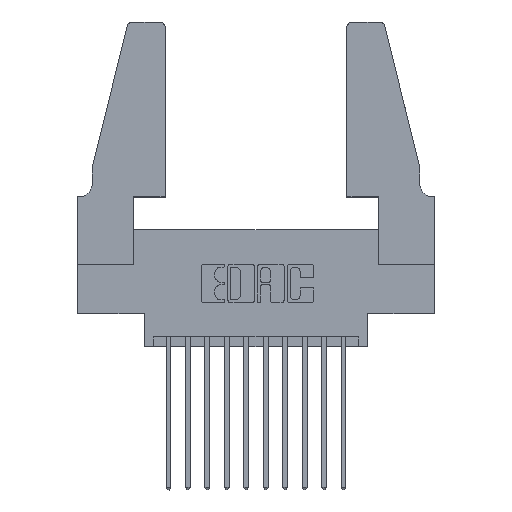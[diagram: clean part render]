
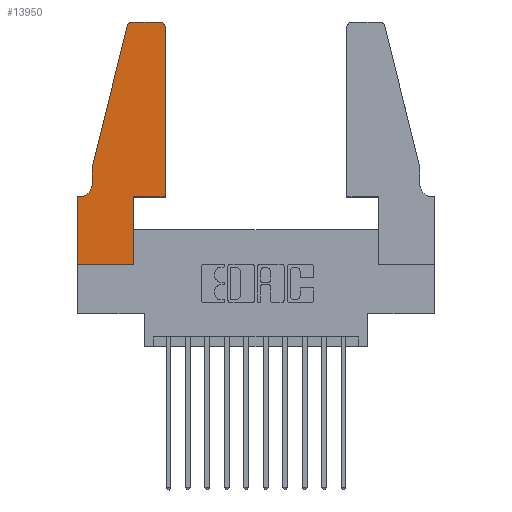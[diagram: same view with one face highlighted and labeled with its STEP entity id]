
A CAD part, top view. The second image highlights one B-rep face of the part: STEP entity #13950.
In plain terms, the highlighted planar face has unit normal (0, 0, 1).
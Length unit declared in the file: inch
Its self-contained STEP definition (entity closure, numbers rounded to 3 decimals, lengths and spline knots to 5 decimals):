
#338 = EDGE_CURVE ( 'NONE', #12182, #7786, #9535, .T. ) ;
#450 = CARTESIAN_POINT ( 'NONE',  ( 0., 0., 0.37 ) ) ;
#765 = VECTOR ( 'NONE', #12722, 39.37008 ) ;
#944 = ORIENTED_EDGE ( 'NONE', *, *, #14025, .T. ) ;
#970 = LINE ( 'NONE', #11142, #13198 ) ;
#1076 = ORIENTED_EDGE ( 'NONE', *, *, #338, .T. ) ;
#1112 = LINE ( 'NONE', #12904, #765 ) ;
#1614 = ORIENTED_EDGE ( 'NONE', *, *, #1717, .T. ) ;
#1717 = EDGE_CURVE ( 'NONE', #2778, #13175, #6778, .T. ) ;
#1848 = CARTESIAN_POINT ( 'NONE',  ( 0.2605, 1.25, 0.37 ) ) ;
#2038 = CARTESIAN_POINT ( 'NONE',  ( 0.0755, 0.5, 0.37 ) ) ;
#2198 = CARTESIAN_POINT ( 'NONE',  ( 0.0755, 0.42, 0.37 ) ) ;
#2309 = VERTEX_POINT ( 'NONE', #2038 ) ;
#2341 = CARTESIAN_POINT ( 'NONE',  ( 0., 0.35, 0.37 ) ) ;
#2718 = DIRECTION ( 'NONE',  ( 0., -1., 0. ) ) ;
#2744 = DIRECTION ( 'NONE',  ( -1., 0., 0. ) ) ;
#2778 = VERTEX_POINT ( 'NONE', #10514 ) ;
#2818 = CARTESIAN_POINT ( 'NONE',  ( 0., 0., 0.37 ) ) ;
#2894 = ORIENTED_EDGE ( 'NONE', *, *, #13201, .T. ) ;
#3040 = VERTEX_POINT ( 'NONE', #12127 ) ;
#3159 = AXIS2_PLACEMENT_3D ( 'NONE', #13959, #9419, #2744 ) ;
#3194 = LINE ( 'NONE', #6531, #11708 ) ;
#3258 = CARTESIAN_POINT ( 'NONE',  ( 0.0055, 0.35, 0.37 ) ) ;
#3302 = DIRECTION ( 'NONE',  ( -1., 0., 0. ) ) ;
#3457 = DIRECTION ( 'NONE',  ( 0., 0., 1. ) ) ;
#3555 = DIRECTION ( 'NONE',  ( 0., 0., 1. ) ) ;
#3777 = DIRECTION ( 'NONE',  ( 1., 0., 0. ) ) ;
#4109 = LINE ( 'NONE', #12534, #6347 ) ;
#4154 = VECTOR ( 'NONE', #7382, 39.37008 ) ;
#4204 = CARTESIAN_POINT ( 'NONE',  ( 0.2865, 0.35, 0.37 ) ) ;
#4251 = LINE ( 'NONE', #450, #8749 ) ;
#4361 = VERTEX_POINT ( 'NONE', #9597 ) ;
#4461 = CARTESIAN_POINT ( 'NONE',  ( 0.25487, 1.22718, 0.37 ) ) ;
#4660 = AXIS2_PLACEMENT_3D ( 'NONE', #10154, #3457, #11219 ) ;
#4676 = EDGE_CURVE ( 'NONE', #10553, #12045, #11576, .T. ) ;
#5004 = FACE_OUTER_BOUND ( 'NONE', #14251, .T. ) ;
#5472 = CARTESIAN_POINT ( 'NONE',  ( 0.284, 1.22, 0.37 ) ) ;
#5544 = ORIENTED_EDGE ( 'NONE', *, *, #4676, .T. ) ;
#5719 = ORIENTED_EDGE ( 'NONE', *, *, #8853, .T. ) ;
#6009 = DIRECTION ( 'NONE',  ( 1., 0., 0. ) ) ;
#6039 = DIRECTION ( 'NONE',  ( 0., -1., 0. ) ) ;
#6179 = VECTOR ( 'NONE', #3777, 39.37008 ) ;
#6347 = VECTOR ( 'NONE', #6039, 39.37008 ) ;
#6531 = CARTESIAN_POINT ( 'NONE',  ( 0.0755, 0.35, 0.37 ) ) ;
#6666 = AXIS2_PLACEMENT_3D ( 'NONE', #2341, #3555, #6862 ) ;
#6708 = DIRECTION ( 'NONE',  ( -0.239, -0.971, 0. ) ) ;
#6778 = CIRCLE ( 'NONE', #11826, 0.03 ) ;
#6862 = DIRECTION ( 'NONE',  ( 1., 0., 0. ) ) ;
#6873 = EDGE_CURVE ( 'NONE', #3040, #7133, #4251, .T. ) ;
#7133 = VERTEX_POINT ( 'NONE', #2818 ) ;
#7382 = DIRECTION ( 'NONE',  ( -1., 0., 0. ) ) ;
#7710 = DIRECTION ( 'NONE',  ( 0., 0., 1. ) ) ;
#7786 = VERTEX_POINT ( 'NONE', #3258 ) ;
#7828 = EDGE_CURVE ( 'NONE', #12045, #11913, #1112, .T. ) ;
#8384 = VERTEX_POINT ( 'NONE', #13131 ) ;
#8546 = LINE ( 'NONE', #1848, #4154 ) ;
#8749 = VECTOR ( 'NONE', #2718, 39.37008 ) ;
#8824 = ORIENTED_EDGE ( 'NONE', *, *, #6873, .T. ) ;
#8853 = EDGE_CURVE ( 'NONE', #2309, #12182, #4109, .T. ) ;
#8856 = ORIENTED_EDGE ( 'NONE', *, *, #9802, .T. ) ;
#9352 = CARTESIAN_POINT ( 'NONE',  ( 0.4505, 0.35, 0.37 ) ) ;
#9419 = DIRECTION ( 'NONE',  ( 0., 0., -1. ) ) ;
#9535 = CIRCLE ( 'NONE', #3159, 0.07 ) ;
#9597 = CARTESIAN_POINT ( 'NONE',  ( 0.4205, 1.25, 0.37 ) ) ;
#9599 = VECTOR ( 'NONE', #14372, 39.37008 ) ;
#9756 = VECTOR ( 'NONE', #14458, 39.37008 ) ;
#9802 = EDGE_CURVE ( 'NONE', #7786, #3040, #3194, .T. ) ;
#10154 = CARTESIAN_POINT ( 'NONE',  ( 0.4205, 1.22, 0.37 ) ) ;
#10514 = CARTESIAN_POINT ( 'NONE',  ( 0.284, 1.25, 0.37 ) ) ;
#10553 = VERTEX_POINT ( 'NONE', #14021 ) ;
#10754 = EDGE_CURVE ( 'NONE', #8384, #10553, #12530, .T. ) ;
#10762 = ORIENTED_EDGE ( 'NONE', *, *, #7828, .T. ) ;
#10914 = ORIENTED_EDGE ( 'NONE', *, *, #12144, .T. ) ;
#11142 = CARTESIAN_POINT ( 'NONE',  ( 0.0755, 0.5, 0.37 ) ) ;
#11219 = DIRECTION ( 'NONE',  ( 1., 0., 0. ) ) ;
#11576 = LINE ( 'NONE', #9352, #6179 ) ;
#11708 = VECTOR ( 'NONE', #3302, 39.37008 ) ;
#11826 = AXIS2_PLACEMENT_3D ( 'NONE', #5472, #7710, #6009 ) ;
#11830 = LINE ( 'NONE', #14369, #9756 ) ;
#11913 = VERTEX_POINT ( 'NONE', #11950 ) ;
#11950 = CARTESIAN_POINT ( 'NONE',  ( 0.4505, 1.22, 0.37 ) ) ;
#11962 = CIRCLE ( 'NONE', #4660, 0.03 ) ;
#12045 = VERTEX_POINT ( 'NONE', #13213 ) ;
#12112 = ORIENTED_EDGE ( 'NONE', *, *, #10754, .T. ) ;
#12127 = CARTESIAN_POINT ( 'NONE',  ( 0., 0.35, 0.37 ) ) ;
#12144 = EDGE_CURVE ( 'NONE', #7133, #8384, #11830, .T. ) ;
#12182 = VERTEX_POINT ( 'NONE', #2198 ) ;
#12298 = ORIENTED_EDGE ( 'NONE', *, *, #13777, .T. ) ;
#12530 = LINE ( 'NONE', #4204, #9599 ) ;
#12534 = CARTESIAN_POINT ( 'NONE',  ( 0.0755, 0.5, 0.37 ) ) ;
#12722 = DIRECTION ( 'NONE',  ( 0., 1., 0. ) ) ;
#12904 = CARTESIAN_POINT ( 'NONE',  ( 0.4505, 0.35, 0.37 ) ) ;
#13131 = CARTESIAN_POINT ( 'NONE',  ( 0.2865, 0., 0.37 ) ) ;
#13175 = VERTEX_POINT ( 'NONE', #4461 ) ;
#13198 = VECTOR ( 'NONE', #6708, 39.37008 ) ;
#13201 = EDGE_CURVE ( 'NONE', #13175, #2309, #970, .T. ) ;
#13213 = CARTESIAN_POINT ( 'NONE',  ( 0.4505, 0.35, 0.37 ) ) ;
#13500 = PLANE ( 'NONE',  #6666 ) ;
#13777 = EDGE_CURVE ( 'NONE', #4361, #2778, #8546, .T. ) ;
#13950 = ADVANCED_FACE ( 'NONE', ( #5004 ), #13500, .T. ) ;
#13959 = CARTESIAN_POINT ( 'NONE',  ( 0.0055, 0.42, 0.37 ) ) ;
#14021 = CARTESIAN_POINT ( 'NONE',  ( 0.2865, 0.35, 0.37 ) ) ;
#14025 = EDGE_CURVE ( 'NONE', #11913, #4361, #11962, .T. ) ;
#14251 = EDGE_LOOP ( 'NONE', ( #12298, #1614, #2894, #5719, #1076, #8856, #8824, #10914, #12112, #5544, #10762, #944 ) ) ;
#14369 = CARTESIAN_POINT ( 'NONE',  ( 0., 0., 0.37 ) ) ;
#14372 = DIRECTION ( 'NONE',  ( 0., 1., 0. ) ) ;
#14458 = DIRECTION ( 'NONE',  ( 1., 0., 0. ) ) ;
